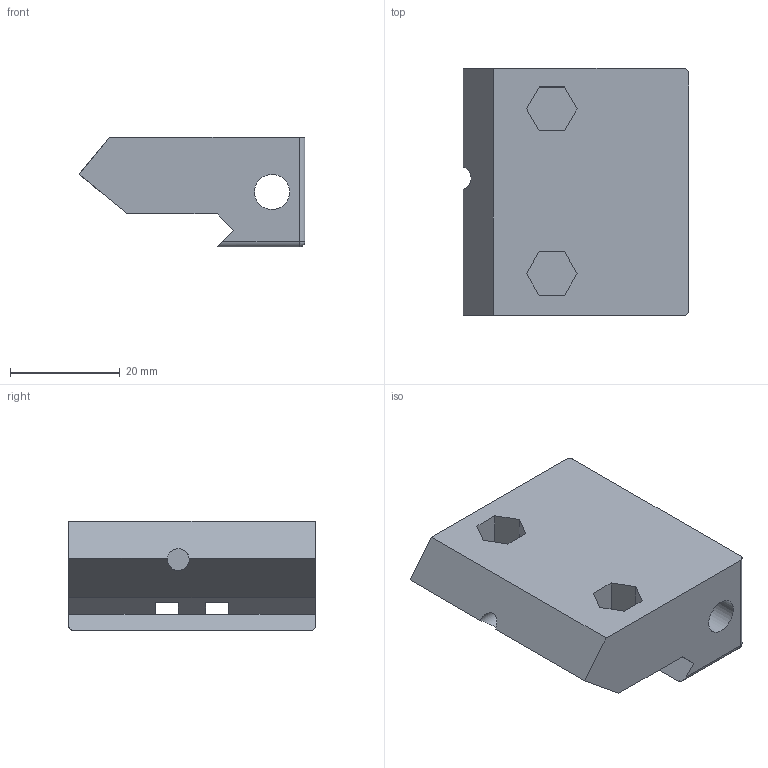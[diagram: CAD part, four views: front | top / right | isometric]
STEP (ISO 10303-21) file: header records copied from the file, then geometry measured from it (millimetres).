
FILE_DESCRIPTION(('FreeCAD Model'),'2;1');
FILE_NAME('V1.1 STL''s & Steps/Right Block V1.1.step','2020-07-30T16:37:58',('Author'),( ''),'Open CASCADE STEP processor 7.3','FreeCAD','Unknown');
FILE_SCHEMA(('AUTOMOTIVE_DESIGN { 1 0 10303 214 1 1 1 1 }'));
Length unit declared in the file: millimetre
Products named in the file (1): Pocket006
Bounding box: 41.17 x 45 x 20 mm (x, y, z)
Volume: 24989.5 mm3; surface area: 8097.8 mm2
Topology: 1 solids, 1 shells, 43 faces, 119 edges, 76 vertices
Faces by surface type: plane 33, cylinder 8, sphere 2
Full cylindrical faces by diameter (mm): 2.5 x1, 4 x1, 6.4 x1
Entity records: 3124 total; most frequent: CARTESIAN_POINT 728, DIRECTION 443, LINE 315, VECTOR 315, ORIENTED_EDGE 234, PCURVE 234, DEFINITIONAL_REPRESENTATION 234, EDGE_CURVE 117
